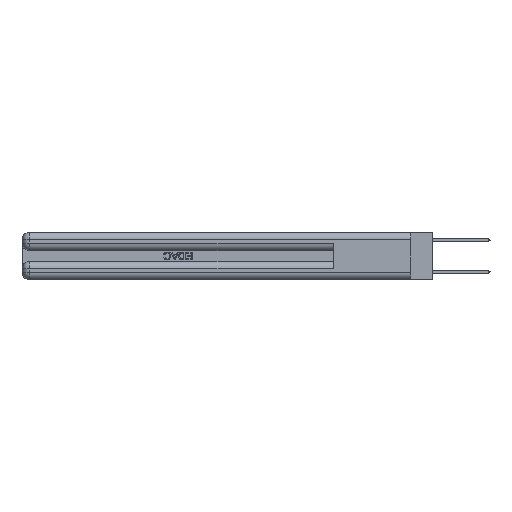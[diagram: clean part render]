
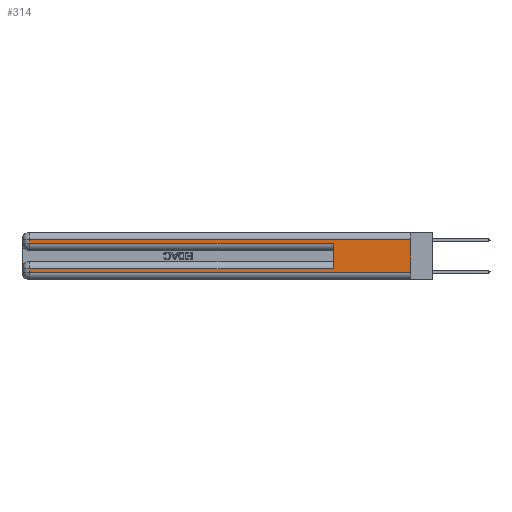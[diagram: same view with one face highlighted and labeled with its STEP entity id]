
A CAD part, left-side view. The second image highlights one B-rep face of the part: STEP entity #314.
In plain terms, the highlighted planar face has unit normal (-1, 0, 0).
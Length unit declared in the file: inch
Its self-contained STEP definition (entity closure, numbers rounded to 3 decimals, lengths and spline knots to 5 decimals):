
#68 = CARTESIAN_POINT ( 'NONE',  ( 0., 0., 0.31 ) ) ;
#177 = EDGE_CURVE ( 'NONE', #11942, #19677, #8306, .T. ) ;
#314 = ADVANCED_FACE ( 'NONE', ( #17493 ), #9150, .F. ) ;
#421 = LINE ( 'NONE', #18513, #16221 ) ;
#1136 = DIRECTION ( 'NONE',  ( 0., 0., 1. ) ) ;
#1641 = AXIS2_PLACEMENT_3D ( 'NONE', #32862, #4341, #4508 ) ;
#1733 = CARTESIAN_POINT ( 'NONE',  ( 0., 2.94, 0.06 ) ) ;
#2216 = VERTEX_POINT ( 'NONE', #15100 ) ;
#2247 = CARTESIAN_POINT ( 'NONE',  ( 0., 0.6, 0.085 ) ) ;
#3646 = VECTOR ( 'NONE', #17335, 39.37008 ) ;
#4341 = DIRECTION ( 'NONE',  ( 1., 0., 0. ) ) ;
#4508 = DIRECTION ( 'NONE',  ( 0., 0., -1. ) ) ;
#4665 = LINE ( 'NONE', #68, #20525 ) ;
#5223 = DIRECTION ( 'NONE',  ( 0., 0., -1. ) ) ;
#5785 = DIRECTION ( 'NONE',  ( 0., -1., 0. ) ) ;
#7573 = CARTESIAN_POINT ( 'NONE',  ( 0., 2.94, 0.37 ) ) ;
#8095 = DIRECTION ( 'NONE',  ( 0., -1., 0. ) ) ;
#8306 = LINE ( 'NONE', #21786, #22366 ) ;
#8873 = ORIENTED_EDGE ( 'NONE', *, *, #24661, .T. ) ;
#9150 = PLANE ( 'NONE',  #1641 ) ;
#10281 = EDGE_CURVE ( 'NONE', #2216, #11492, #4665, .T. ) ;
#10334 = ORIENTED_EDGE ( 'NONE', *, *, #24491, .F. ) ;
#10650 = DIRECTION ( 'NONE',  ( 0., 0., -1. ) ) ;
#11492 = VERTEX_POINT ( 'NONE', #22099 ) ;
#11690 = VERTEX_POINT ( 'NONE', #31647 ) ;
#11942 = VERTEX_POINT ( 'NONE', #2247 ) ;
#13434 = LINE ( 'NONE', #18542, #19571 ) ;
#13660 = LINE ( 'NONE', #14002, #20832 ) ;
#14002 = CARTESIAN_POINT ( 'NONE',  ( 0., 0., 0.06 ) ) ;
#14324 = VERTEX_POINT ( 'NONE', #1733 ) ;
#15100 = CARTESIAN_POINT ( 'NONE',  ( 0., 0., 0.31 ) ) ;
#15292 = LINE ( 'NONE', #30490, #3646 ) ;
#15773 = LINE ( 'NONE', #7573, #20931 ) ;
#16043 = ORIENTED_EDGE ( 'NONE', *, *, #21109, .T. ) ;
#16221 = VECTOR ( 'NONE', #8095, 39.37008 ) ;
#16318 = EDGE_CURVE ( 'NONE', #11942, #30388, #16706, .T. ) ;
#16706 = LINE ( 'NONE', #27127, #23994 ) ;
#17335 = DIRECTION ( 'NONE',  ( 0., 0., -1. ) ) ;
#17493 = FACE_OUTER_BOUND ( 'NONE', #30369, .T. ) ;
#18513 = CARTESIAN_POINT ( 'NONE',  ( 0., 0., 0.285 ) ) ;
#18542 = CARTESIAN_POINT ( 'NONE',  ( 0., 2.94, 0.37 ) ) ;
#19571 = VECTOR ( 'NONE', #5223, 39.37008 ) ;
#19677 = VERTEX_POINT ( 'NONE', #25511 ) ;
#20525 = VECTOR ( 'NONE', #25512, 39.37008 ) ;
#20832 = VECTOR ( 'NONE', #5785, 39.37008 ) ;
#20931 = VECTOR ( 'NONE', #10650, 39.37008 ) ;
#21109 = EDGE_CURVE ( 'NONE', #11492, #27102, #15773, .T. ) ;
#21299 = DIRECTION ( 'NONE',  ( 0., 1., 0. ) ) ;
#21786 = CARTESIAN_POINT ( 'NONE',  ( 0., 0.6, 0.145 ) ) ;
#22099 = CARTESIAN_POINT ( 'NONE',  ( 0., 2.94, 0.31 ) ) ;
#22366 = VECTOR ( 'NONE', #1136, 39.37008 ) ;
#23994 = VECTOR ( 'NONE', #21299, 39.37008 ) ;
#24491 = EDGE_CURVE ( 'NONE', #2216, #11690, #15292, .T. ) ;
#24661 = EDGE_CURVE ( 'NONE', #27102, #19677, #421, .T. ) ;
#25511 = CARTESIAN_POINT ( 'NONE',  ( 0., 0.6, 0.285 ) ) ;
#25512 = DIRECTION ( 'NONE',  ( 0., 1., 0. ) ) ;
#26443 = CARTESIAN_POINT ( 'NONE',  ( 0., 2.94, 0.285 ) ) ;
#27102 = VERTEX_POINT ( 'NONE', #26443 ) ;
#27127 = CARTESIAN_POINT ( 'NONE',  ( 0., 0., 0.085 ) ) ;
#27799 = CARTESIAN_POINT ( 'NONE',  ( 0., 2.94, 0.085 ) ) ;
#28523 = ORIENTED_EDGE ( 'NONE', *, *, #16318, .T. ) ;
#28765 = EDGE_CURVE ( 'NONE', #30388, #14324, #13434, .T. ) ;
#30369 = EDGE_LOOP ( 'NONE', ( #10334, #32390, #16043, #8873, #32084, #28523, #31746, #33455 ) ) ;
#30388 = VERTEX_POINT ( 'NONE', #27799 ) ;
#30490 = CARTESIAN_POINT ( 'NONE',  ( 0., 0., 0.37 ) ) ;
#31647 = CARTESIAN_POINT ( 'NONE',  ( 0., 0., 0.06 ) ) ;
#31746 = ORIENTED_EDGE ( 'NONE', *, *, #28765, .T. ) ;
#32084 = ORIENTED_EDGE ( 'NONE', *, *, #177, .F. ) ;
#32390 = ORIENTED_EDGE ( 'NONE', *, *, #10281, .T. ) ;
#32651 = EDGE_CURVE ( 'NONE', #14324, #11690, #13660, .T. ) ;
#32862 = CARTESIAN_POINT ( 'NONE',  ( 0., 0., 0.37 ) ) ;
#33455 = ORIENTED_EDGE ( 'NONE', *, *, #32651, .T. ) ;
